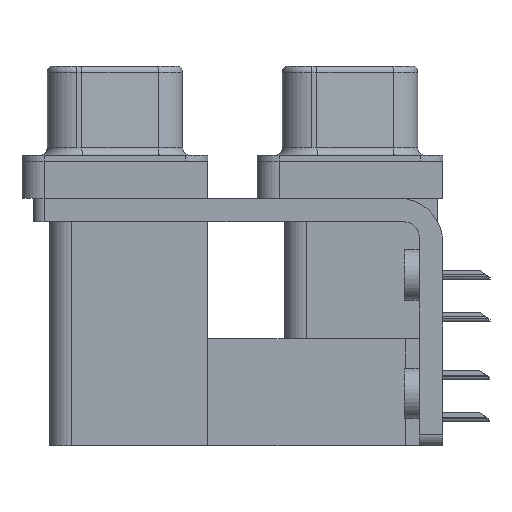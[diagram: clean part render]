
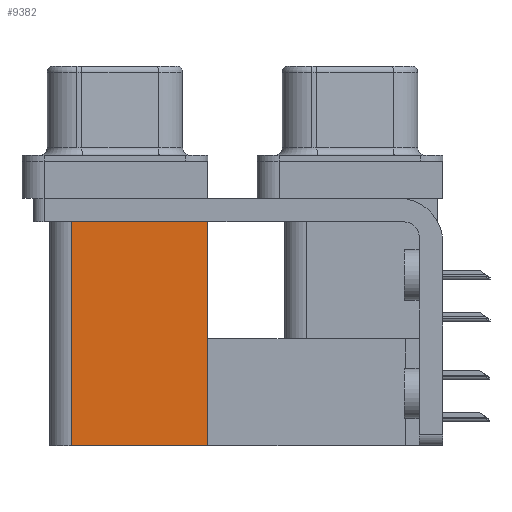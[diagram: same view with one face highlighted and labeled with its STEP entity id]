
A CAD part, left-side view. The second image highlights one B-rep face of the part: STEP entity #9382.
In plain terms, the highlighted planar face has unit normal (-1, 0, 0).
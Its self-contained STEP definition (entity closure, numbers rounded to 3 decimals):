
#374 = DIRECTION ( 'NONE',  ( 0., 0., -1. ) ) ;
#774 = CARTESIAN_POINT ( 'NONE',  ( 3.7, 9.6, -19.2 ) ) ;
#980 = DIRECTION ( 'NONE',  ( 1., 0., 0. ) ) ;
#6650 = EDGE_LOOP ( 'NONE', ( #11167, #17390, #36817, #8464 ) ) ;
#6672 = FACE_OUTER_BOUND ( 'NONE', #6650, .T. ) ;
#7174 = VECTOR ( 'NONE', #26035, 1000. ) ;
#7661 = CARTESIAN_POINT ( 'NONE',  ( 3.7, 9.6, -19.2 ) ) ;
#8464 = ORIENTED_EDGE ( 'NONE', *, *, #21650, .T. ) ;
#8952 = LINE ( 'NONE', #14862, #28292 ) ;
#9382 = ADVANCED_FACE ( 'NONE', ( #6672 ), #35274, .F. ) ;
#9423 = CARTESIAN_POINT ( 'NONE',  ( 3.7, 18.8, -19.2 ) ) ;
#11167 = ORIENTED_EDGE ( 'NONE', *, *, #30206, .T. ) ;
#14272 = VERTEX_POINT ( 'NONE', #34415 ) ;
#14862 = CARTESIAN_POINT ( 'NONE',  ( 3.7, 9.6, -2.5 ) ) ;
#14877 = DIRECTION ( 'NONE',  ( 0., 0., 1. ) ) ;
#15926 = DIRECTION ( 'NONE',  ( 0., 0., 1. ) ) ;
#17153 = VERTEX_POINT ( 'NONE', #40247 ) ;
#17390 = ORIENTED_EDGE ( 'NONE', *, *, #36930, .F. ) ;
#17717 = CARTESIAN_POINT ( 'NONE',  ( 3.7, 18.8, -2.5 ) ) ;
#18999 = LINE ( 'NONE', #9423, #22241 ) ;
#19962 = VERTEX_POINT ( 'NONE', #32476 ) ;
#21400 = DIRECTION ( 'NONE',  ( 0., 1., 0. ) ) ;
#21650 = EDGE_CURVE ( 'NONE', #17153, #14272, #28158, .T. ) ;
#22241 = VECTOR ( 'NONE', #15926, 1000. ) ;
#26035 = DIRECTION ( 'NONE',  ( 0., 1., 0. ) ) ;
#27550 = CARTESIAN_POINT ( 'NONE',  ( 3.7, 9.6, -19.2 ) ) ;
#27886 = EDGE_CURVE ( 'NONE', #17153, #19962, #32579, .T. ) ;
#28158 = LINE ( 'NONE', #27550, #36901 ) ;
#28292 = VECTOR ( 'NONE', #21400, 1000. ) ;
#30206 = EDGE_CURVE ( 'NONE', #14272, #32380, #8952, .T. ) ;
#32380 = VERTEX_POINT ( 'NONE', #17717 ) ;
#32476 = CARTESIAN_POINT ( 'NONE',  ( 3.7, 18.8, -19.2 ) ) ;
#32579 = LINE ( 'NONE', #7661, #7174 ) ;
#33565 = AXIS2_PLACEMENT_3D ( 'NONE', #774, #980, #374 ) ;
#34415 = CARTESIAN_POINT ( 'NONE',  ( 3.7, 9.6, -2.5 ) ) ;
#35274 = PLANE ( 'NONE',  #33565 ) ;
#36817 = ORIENTED_EDGE ( 'NONE', *, *, #27886, .F. ) ;
#36901 = VECTOR ( 'NONE', #14877, 1000. ) ;
#36930 = EDGE_CURVE ( 'NONE', #19962, #32380, #18999, .T. ) ;
#40247 = CARTESIAN_POINT ( 'NONE',  ( 3.7, 9.6, -19.2 ) ) ;
